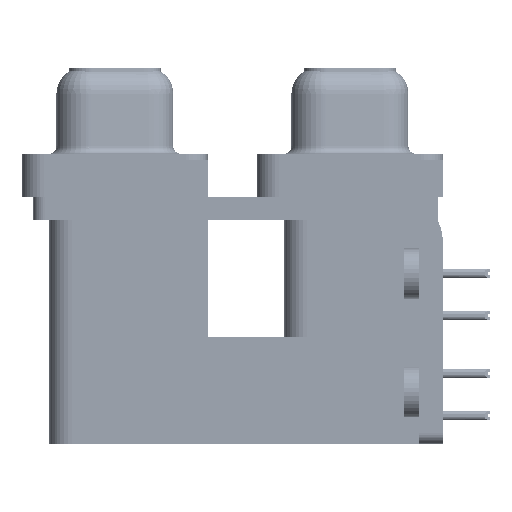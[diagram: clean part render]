
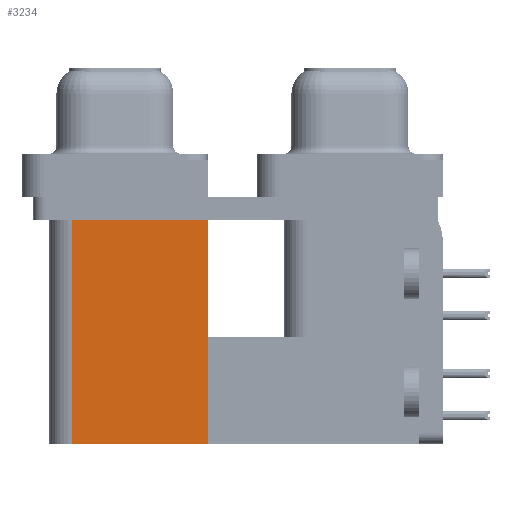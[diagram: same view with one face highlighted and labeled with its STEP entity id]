
A CAD part, left-side view. The second image highlights one B-rep face of the part: STEP entity #3234.
In plain terms, the highlighted planar face has unit normal (-1, 0, 0).
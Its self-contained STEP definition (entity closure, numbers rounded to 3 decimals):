
#569 = CARTESIAN_POINT ( 'NONE',  ( 3.7, 9.6, -19.2 ) ) ;
#644 = LINE ( 'NONE', #15036, #48629 ) ;
#3234 = ADVANCED_FACE ( 'NONE', ( #39476 ), #38284, .F. ) ;
#3566 = EDGE_CURVE ( 'NONE', #42747, #19149, #55973, .T. ) ;
#3741 = VECTOR ( 'NONE', #49984, 1000. ) ;
#4395 = AXIS2_PLACEMENT_3D ( 'NONE', #6145, #20522, #19914 ) ;
#4943 = ORIENTED_EDGE ( 'NONE', *, *, #34679, .F. ) ;
#5618 = VECTOR ( 'NONE', #19264, 1000. ) ;
#6145 = CARTESIAN_POINT ( 'NONE',  ( 3.7, 9.6, -19.2 ) ) ;
#6236 = ORIENTED_EDGE ( 'NONE', *, *, #3566, .T. ) ;
#7988 = EDGE_CURVE ( 'NONE', #19149, #53924, #44794, .T. ) ;
#11547 = CARTESIAN_POINT ( 'NONE',  ( 3.7, 18.8, -19.2 ) ) ;
#15036 = CARTESIAN_POINT ( 'NONE',  ( 3.7, 9.6, -19.2 ) ) ;
#16478 = DIRECTION ( 'NONE',  ( 0., 0., 1. ) ) ;
#19149 = VERTEX_POINT ( 'NONE', #45701 ) ;
#19264 = DIRECTION ( 'NONE',  ( 0., 0., 1. ) ) ;
#19914 = DIRECTION ( 'NONE',  ( 0., 1., 0. ) ) ;
#19915 = DIRECTION ( 'NONE',  ( 0., 1., 0. ) ) ;
#20522 = DIRECTION ( 'NONE',  ( 1., 0., 0. ) ) ;
#24342 = ORIENTED_EDGE ( 'NONE', *, *, #35180, .F. ) ;
#29127 = VERTEX_POINT ( 'NONE', #54129 ) ;
#30531 = LINE ( 'NONE', #11547, #35870 ) ;
#31332 = CARTESIAN_POINT ( 'NONE',  ( 3.7, 9.6, -2.5 ) ) ;
#33000 = CARTESIAN_POINT ( 'NONE',  ( 3.7, 18.8, -2.5 ) ) ;
#34679 = EDGE_CURVE ( 'NONE', #29127, #53924, #30531, .T. ) ;
#35180 = EDGE_CURVE ( 'NONE', #42747, #29127, #644, .T. ) ;
#35870 = VECTOR ( 'NONE', #16478, 1000. ) ;
#38284 = PLANE ( 'NONE',  #4395 ) ;
#39476 = FACE_OUTER_BOUND ( 'NONE', #60017, .T. ) ;
#42279 = ORIENTED_EDGE ( 'NONE', *, *, #7988, .T. ) ;
#42747 = VERTEX_POINT ( 'NONE', #48112 ) ;
#44794 = LINE ( 'NONE', #31332, #3741 ) ;
#45701 = CARTESIAN_POINT ( 'NONE',  ( 3.7, 9.6, -2.5 ) ) ;
#48112 = CARTESIAN_POINT ( 'NONE',  ( 3.7, 9.6, -19.2 ) ) ;
#48629 = VECTOR ( 'NONE', #19915, 1000. ) ;
#49984 = DIRECTION ( 'NONE',  ( 0., 1., 0. ) ) ;
#53924 = VERTEX_POINT ( 'NONE', #33000 ) ;
#54129 = CARTESIAN_POINT ( 'NONE',  ( 3.7, 18.8, -19.2 ) ) ;
#55973 = LINE ( 'NONE', #569, #5618 ) ;
#60017 = EDGE_LOOP ( 'NONE', ( #42279, #4943, #24342, #6236 ) ) ;
